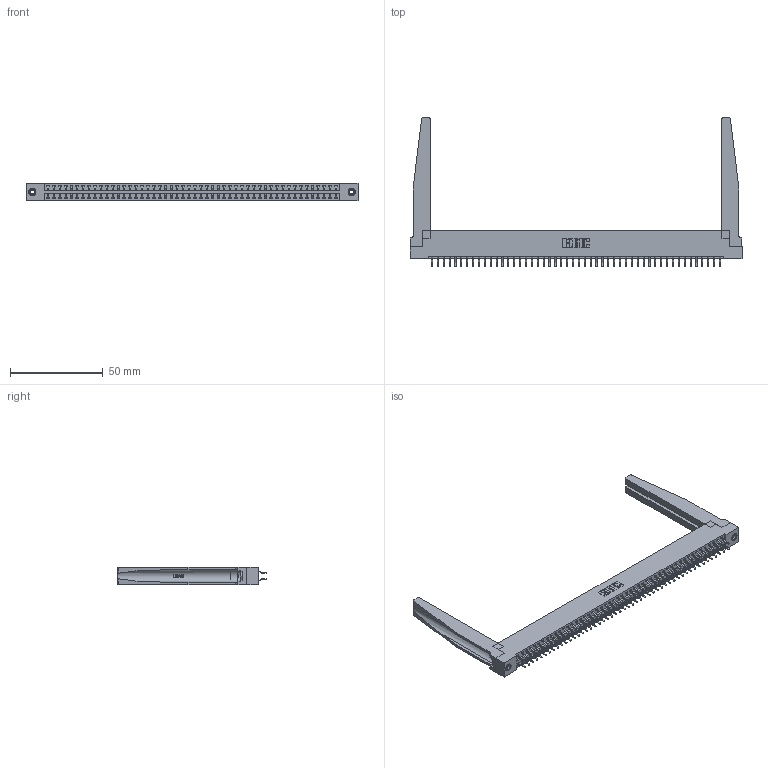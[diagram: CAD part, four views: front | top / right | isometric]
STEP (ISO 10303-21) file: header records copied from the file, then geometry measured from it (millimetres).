
FILE_DESCRIPTION (( 'STEP AP203' ), '1' );
FILE_NAME ('396-100-556-278.STEP', '2019-10-31T06:01:16', ( '' ), ( '' ), 'SwSTEP 2.0', 'SolidWorks 2016', '' );
FILE_SCHEMA (( 'CONFIG_CONTROL_DESIGN' ));
Length unit declared in the file: inch
Products named in the file (5): 396-100-556-278; 346-220-078_345-220-078; 345-292-001_556 Tail; 346 Part_Flush Mounting Lugs - 0.156 Dia-TH; 345-250-001_345-250-001-102
Assembly tree (105 placements, depth 2):
  396-100-556-278
    346 Part_Flush Mounting Lugs - 0.156 Dia-TH
    345-292-001_556 Tail  x100
    346-220-078_345-220-078  x2
    345-250-001_345-250-001-102  x2
Bounding box: 179.32 x 80.53 x 9.4 mm (x, y, z)
Volume: 24453.3 mm3; surface area: 30686.4 mm2
Topology: 105 solids, 105 shells, 6156 faces, 18237 edges, 12014 vertices
Faces by surface type: plane 4118, cylinder 1986, bspline 36, cone 12, torus 4
Entity records: 36522 total; most frequent: CARTESIAN_POINT 6959, ORIENTED_EDGE 5770, DIRECTION 5159, EDGE_CURVE 2885, VECTOR 2451, LINE 2451, VERTEX_POINT 1916, AXIS2_PLACEMENT_3D 1354
